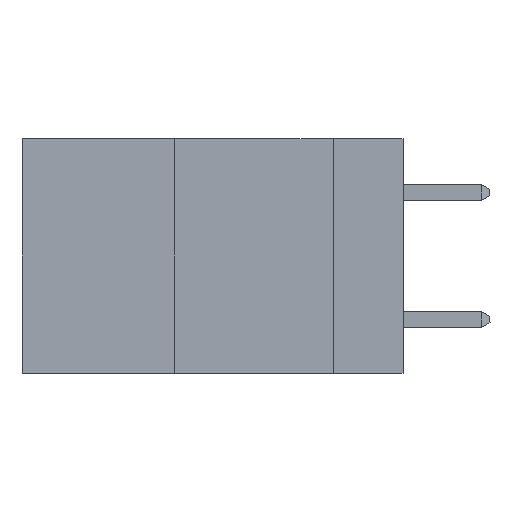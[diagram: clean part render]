
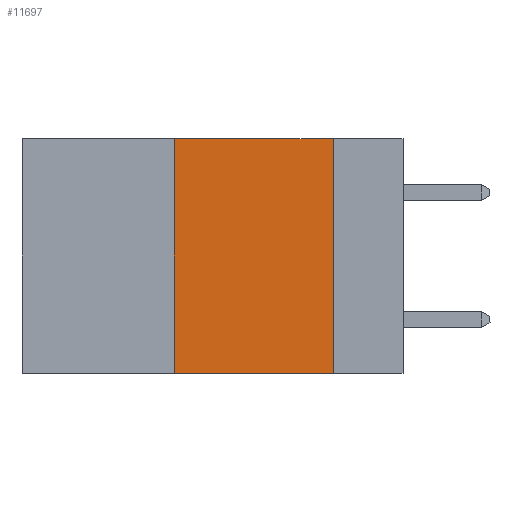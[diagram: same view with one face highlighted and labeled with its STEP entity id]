
A CAD part, left-side view. The second image highlights one B-rep face of the part: STEP entity #11697.
In plain terms, the highlighted planar face has unit normal (-1, 0, 0).
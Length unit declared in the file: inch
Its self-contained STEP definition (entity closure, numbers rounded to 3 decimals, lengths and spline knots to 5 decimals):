
#191 = EDGE_LOOP ( 'NONE', ( #13144, #13106, #12968, #11890 ) ) ;
#400 = VECTOR ( 'NONE', #7624, 39.37008 ) ;
#1092 = EDGE_CURVE ( 'NONE', #11179, #4233, #4157, .T. ) ;
#1157 = CARTESIAN_POINT ( 'NONE',  ( 0., 0.6, 0. ) ) ;
#2714 = DIRECTION ( 'NONE',  ( 0., 0., -1. ) ) ;
#2791 = DIRECTION ( 'NONE',  ( 0., -1., 0. ) ) ;
#3977 = CARTESIAN_POINT ( 'NONE',  ( 0., 0.6, 0. ) ) ;
#4099 = AXIS2_PLACEMENT_3D ( 'NONE', #1157, #11022, #2714 ) ;
#4157 = LINE ( 'NONE', #13440, #8748 ) ;
#4233 = VERTEX_POINT ( 'NONE', #13399 ) ;
#4726 = FACE_OUTER_BOUND ( 'NONE', #191, .T. ) ;
#4867 = EDGE_CURVE ( 'NONE', #18056, #4233, #16704, .T. ) ;
#4908 = VERTEX_POINT ( 'NONE', #7129 ) ;
#4955 = EDGE_CURVE ( 'NONE', #4908, #18056, #15397, .T. ) ;
#7129 = CARTESIAN_POINT ( 'NONE',  ( 0., 0.36, 0. ) ) ;
#7624 = DIRECTION ( 'NONE',  ( 0., -1., 0. ) ) ;
#8715 = DIRECTION ( 'NONE',  ( 0., 0., -1. ) ) ;
#8748 = VECTOR ( 'NONE', #2791, 39.37008 ) ;
#9148 = CARTESIAN_POINT ( 'NONE',  ( 0., 0.11, 0. ) ) ;
#9453 = VECTOR ( 'NONE', #8715, 39.37008 ) ;
#9704 = PLANE ( 'NONE',  #4099 ) ;
#11022 = DIRECTION ( 'NONE',  ( 1., 0., 0. ) ) ;
#11179 = VERTEX_POINT ( 'NONE', #15667 ) ;
#11697 = ADVANCED_FACE ( 'NONE', ( #4726 ), #9704, .F. ) ;
#11890 = ORIENTED_EDGE ( 'NONE', *, *, #1092, .T. ) ;
#12652 = DIRECTION ( 'NONE',  ( 0., 0., 1. ) ) ;
#12968 = ORIENTED_EDGE ( 'NONE', *, *, #13672, .F. ) ;
#13106 = ORIENTED_EDGE ( 'NONE', *, *, #4955, .F. ) ;
#13144 = ORIENTED_EDGE ( 'NONE', *, *, #4867, .F. ) ;
#13227 = VECTOR ( 'NONE', #12652, 39.37008 ) ;
#13399 = CARTESIAN_POINT ( 'NONE',  ( 0., 0.11, -0.37 ) ) ;
#13440 = CARTESIAN_POINT ( 'NONE',  ( 0., 0.6, -0.37 ) ) ;
#13672 = EDGE_CURVE ( 'NONE', #11179, #4908, #16883, .T. ) ;
#13968 = CARTESIAN_POINT ( 'NONE',  ( 0., 0.36, 0. ) ) ;
#15397 = LINE ( 'NONE', #3977, #400 ) ;
#15667 = CARTESIAN_POINT ( 'NONE',  ( 0., 0.36, -0.37 ) ) ;
#16704 = LINE ( 'NONE', #9148, #9453 ) ;
#16883 = LINE ( 'NONE', #13968, #13227 ) ;
#16987 = CARTESIAN_POINT ( 'NONE',  ( 0., 0.11, 0. ) ) ;
#18056 = VERTEX_POINT ( 'NONE', #16987 ) ;
